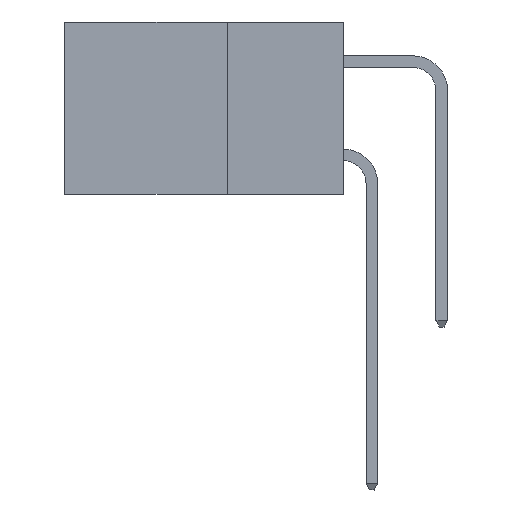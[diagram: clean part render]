
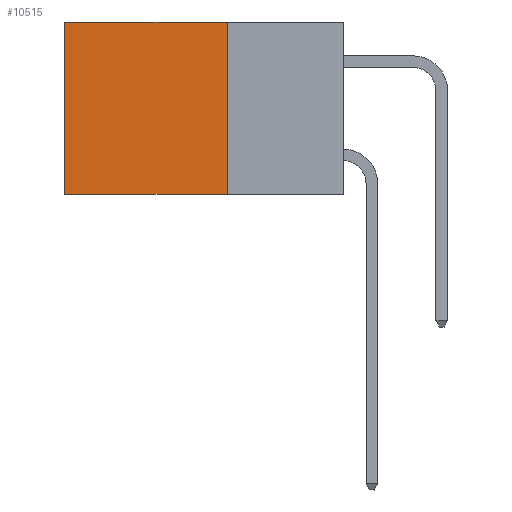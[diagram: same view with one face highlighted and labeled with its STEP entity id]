
A CAD part, left-side view. The second image highlights one B-rep face of the part: STEP entity #10515.
In plain terms, the highlighted planar face has unit normal (-1, 0, 0).
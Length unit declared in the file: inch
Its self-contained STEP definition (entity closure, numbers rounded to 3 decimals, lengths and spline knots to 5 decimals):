
#151 = DIRECTION ( 'NONE',  ( 1., 0., 0. ) ) ;
#362 = VERTEX_POINT ( 'NONE', #7354 ) ;
#877 = CARTESIAN_POINT ( 'NONE',  ( 0.2615, 0.25, -0.37 ) ) ;
#1087 = ORIENTED_EDGE ( 'NONE', *, *, #7787, .T. ) ;
#1711 = DIRECTION ( 'NONE',  ( 0., 1., 0. ) ) ;
#1871 = PLANE ( 'NONE',  #5846 ) ;
#2220 = LINE ( 'NONE', #2549, #12321 ) ;
#2549 = CARTESIAN_POINT ( 'NONE',  ( 0.2615, 0.25, -0.37 ) ) ;
#2622 = VECTOR ( 'NONE', #7168, 39.37008 ) ;
#3113 = VERTEX_POINT ( 'NONE', #6209 ) ;
#4790 = DIRECTION ( 'NONE',  ( 0., 1., 0. ) ) ;
#5086 = EDGE_LOOP ( 'NONE', ( #1087, #11487, #8999, #10557 ) ) ;
#5844 = LINE ( 'NONE', #8033, #8743 ) ;
#5846 = AXIS2_PLACEMENT_3D ( 'NONE', #877, #151, #10981 ) ;
#6209 = CARTESIAN_POINT ( 'NONE',  ( 0.2615, 0.6, 0. ) ) ;
#6395 = CARTESIAN_POINT ( 'NONE',  ( 0.2615, 0.25, -0.37 ) ) ;
#6516 = VECTOR ( 'NONE', #1711, 39.37008 ) ;
#6537 = VERTEX_POINT ( 'NONE', #7890 ) ;
#7168 = DIRECTION ( 'NONE',  ( 0., 0., -1. ) ) ;
#7354 = CARTESIAN_POINT ( 'NONE',  ( 0.2615, 0.6, -0.37 ) ) ;
#7574 = EDGE_CURVE ( 'NONE', #12564, #362, #2220, .T. ) ;
#7787 = EDGE_CURVE ( 'NONE', #3113, #362, #5844, .T. ) ;
#7890 = CARTESIAN_POINT ( 'NONE',  ( 0.2615, 0.25, 0. ) ) ;
#7957 = EDGE_CURVE ( 'NONE', #6537, #12564, #8418, .T. ) ;
#8033 = CARTESIAN_POINT ( 'NONE',  ( 0.2615, 0.6, -0.37 ) ) ;
#8153 = CARTESIAN_POINT ( 'NONE',  ( 0.2615, 0.25, -0.37 ) ) ;
#8418 = LINE ( 'NONE', #8153, #2622 ) ;
#8743 = VECTOR ( 'NONE', #11987, 39.37008 ) ;
#8999 = ORIENTED_EDGE ( 'NONE', *, *, #7957, .F. ) ;
#10515 = ADVANCED_FACE ( 'NONE', ( #10905 ), #1871, .F. ) ;
#10557 = ORIENTED_EDGE ( 'NONE', *, *, #11240, .T. ) ;
#10747 = CARTESIAN_POINT ( 'NONE',  ( 0.2615, 0.25, 0. ) ) ;
#10905 = FACE_OUTER_BOUND ( 'NONE', #5086, .T. ) ;
#10981 = DIRECTION ( 'NONE',  ( 0., 0., -1. ) ) ;
#11240 = EDGE_CURVE ( 'NONE', #6537, #3113, #11620, .T. ) ;
#11487 = ORIENTED_EDGE ( 'NONE', *, *, #7574, .F. ) ;
#11620 = LINE ( 'NONE', #10747, #6516 ) ;
#11987 = DIRECTION ( 'NONE',  ( 0., 0., -1. ) ) ;
#12321 = VECTOR ( 'NONE', #4790, 39.37008 ) ;
#12564 = VERTEX_POINT ( 'NONE', #6395 ) ;
